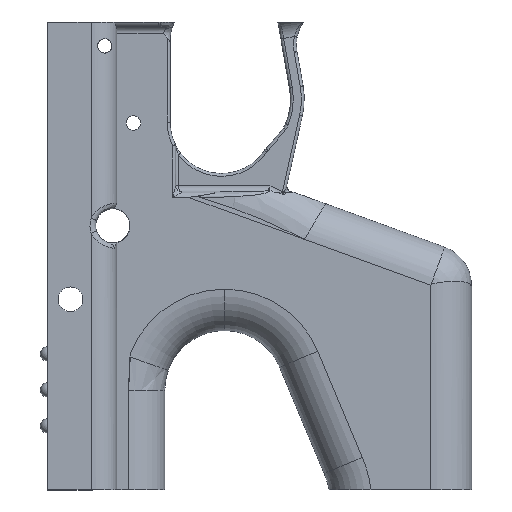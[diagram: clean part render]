
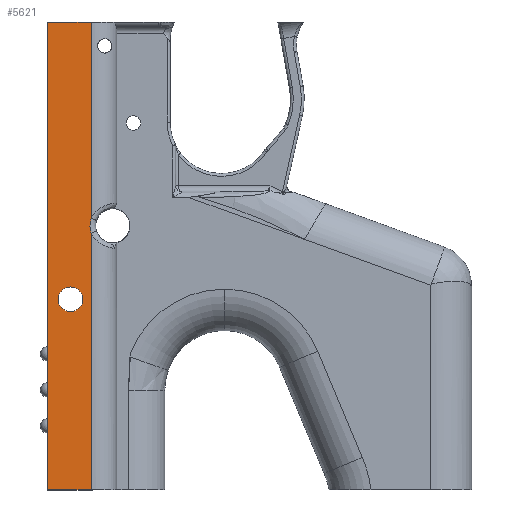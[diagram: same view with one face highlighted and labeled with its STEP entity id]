
A CAD part, left-side view. The second image highlights one B-rep face of the part: STEP entity #5621.
In plain terms, the highlighted planar face has unit normal (-1, 0, 0).
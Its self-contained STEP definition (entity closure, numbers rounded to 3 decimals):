
#21 = VECTOR ( 'NONE', #8800, 1000. ) ;
#68 = EDGE_CURVE ( 'NONE', #7060, #8073, #7952, .T. ) ;
#124 = DIRECTION ( 'NONE',  ( 0., 1., 0. ) ) ;
#207 = DIRECTION ( 'NONE',  ( -1., 0., 0. ) ) ;
#479 = CARTESIAN_POINT ( 'NONE',  ( 4.253, 33.602, 77.663 ) ) ;
#769 = CIRCLE ( 'NONE', #2056, 3.429 ) ;
#933 = VERTEX_POINT ( 'NONE', #3870 ) ;
#952 = CARTESIAN_POINT ( 'NONE',  ( 4.253, 33.602, -52.337 ) ) ;
#1042 = ORIENTED_EDGE ( 'NONE', *, *, #3121, .T. ) ;
#1100 = ORIENTED_EDGE ( 'NONE', *, *, #10105, .F. ) ;
#1214 = ORIENTED_EDGE ( 'NONE', *, *, #10980, .F. ) ;
#1591 = ORIENTED_EDGE ( 'NONE', *, *, #2117, .F. ) ;
#1662 = VERTEX_POINT ( 'NONE', #5119 ) ;
#1721 = CIRCLE ( 'NONE', #8557, 3.429 ) ;
#1729 = CARTESIAN_POINT ( 'NONE',  ( 4.253, 33.602, -52.337 ) ) ;
#1735 = EDGE_CURVE ( 'NONE', #11558, #3343, #9408, .T. ) ;
#2056 = AXIS2_PLACEMENT_3D ( 'NONE', #4003, #10663, #5003 ) ;
#2109 = LINE ( 'NONE', #952, #11608 ) ;
#2117 = EDGE_CURVE ( 'NONE', #1662, #4378, #1721, .T. ) ;
#2332 = AXIS2_PLACEMENT_3D ( 'NONE', #10855, #207, #7182 ) ;
#2620 = CARTESIAN_POINT ( 'NONE',  ( 4.253, 33.602, 19.005 ) ) ;
#2871 = VERTEX_POINT ( 'NONE', #2992 ) ;
#2992 = CARTESIAN_POINT ( 'NONE',  ( 4.253, 45.721, -52.337 ) ) ;
#3102 = EDGE_CURVE ( 'NONE', #7060, #2871, #2109, .T. ) ;
#3121 = EDGE_CURVE ( 'NONE', #8073, #933, #10884, .T. ) ;
#3182 = EDGE_CURVE ( 'NONE', #933, #11558, #9022, .T. ) ;
#3343 = VERTEX_POINT ( 'NONE', #8854 ) ;
#3510 = CARTESIAN_POINT ( 'NONE',  ( 4.253, 33.602, 19.005 ) ) ;
#3870 = CARTESIAN_POINT ( 'NONE',  ( 4.253, 33.602, 23.07 ) ) ;
#4003 = CARTESIAN_POINT ( 'NONE',  ( 4.253, 39.359, 0.641 ) ) ;
#4378 = VERTEX_POINT ( 'NONE', #8688 ) ;
#4851 = CARTESIAN_POINT ( 'NONE',  ( 4.253, 33.602, 77.663 ) ) ;
#5003 = DIRECTION ( 'NONE',  ( 0., 0., 1. ) ) ;
#5119 = CARTESIAN_POINT ( 'NONE',  ( 4.253, 39.359, -2.788 ) ) ;
#5426 = DIRECTION ( 'NONE',  ( 0., 0., 1. ) ) ;
#5463 = ORIENTED_EDGE ( 'NONE', *, *, #3182, .T. ) ;
#5621 = ADVANCED_FACE ( 'NONE', ( #10233, #7756 ), #9979, .T. ) ;
#6222 = CARTESIAN_POINT ( 'NONE',  ( 4.253, 33.602, 141.062 ) ) ;
#6896 = ORIENTED_EDGE ( 'NONE', *, *, #68, .T. ) ;
#7060 = VERTEX_POINT ( 'NONE', #1729 ) ;
#7182 = DIRECTION ( 'NONE',  ( 0., 0., 1. ) ) ;
#7756 = FACE_BOUND ( 'NONE', #11450, .T. ) ;
#7952 = LINE ( 'NONE', #9132, #21 ) ;
#8073 = VERTEX_POINT ( 'NONE', #2620 ) ;
#8542 = DIRECTION ( 'NONE',  ( 0., 0., 1. ) ) ;
#8553 = DIRECTION ( 'NONE',  ( -1., 0., 0. ) ) ;
#8555 = CARTESIAN_POINT ( 'NONE',  ( 4.253, 39.359, 0.641 ) ) ;
#8557 = AXIS2_PLACEMENT_3D ( 'NONE', #8555, #8553, #8542 ) ;
#8688 = CARTESIAN_POINT ( 'NONE',  ( 4.253, 39.359, 4.07 ) ) ;
#8705 = CARTESIAN_POINT ( 'NONE',  ( 4.253, 45.721, 162.566 ) ) ;
#8800 = DIRECTION ( 'NONE',  ( 0., 0., 1. ) ) ;
#8854 = CARTESIAN_POINT ( 'NONE',  ( 4.253, 45.721, 77.663 ) ) ;
#8971 = EDGE_LOOP ( 'NONE', ( #10931, #6896, #1042, #5463, #9931, #1214 ) ) ;
#9022 = LINE ( 'NONE', #6222, #11117 ) ;
#9132 = CARTESIAN_POINT ( 'NONE',  ( 4.253, 33.602, 141.062 ) ) ;
#9408 = LINE ( 'NONE', #4851, #11431 ) ;
#9931 = ORIENTED_EDGE ( 'NONE', *, *, #1735, .T. ) ;
#9979 = PLANE ( 'NONE',  #2332 ) ;
#10105 = EDGE_CURVE ( 'NONE', #4378, #1662, #769, .T. ) ;
#10233 = FACE_OUTER_BOUND ( 'NONE', #8971, .T. ) ;
#10497 = DIRECTION ( 'NONE',  ( 0., 0., 1. ) ) ;
#10565 = DIRECTION ( 'NONE',  ( 0., 1., 0. ) ) ;
#10648 = VECTOR ( 'NONE', #10497, 1000. ) ;
#10663 = DIRECTION ( 'NONE',  ( -1., 0., 0. ) ) ;
#10855 = CARTESIAN_POINT ( 'NONE',  ( 4.253, 33.602, 141.062 ) ) ;
#10884 = B_SPLINE_CURVE_WITH_KNOTS ( 'NONE', 3,
 ( #3510, #11804, #11771, #11738, #11703, #11668 ),
 .UNSPECIFIED., .F., .F.,
 ( 4, 2, 4 ),
 ( 0., 0.5, 1. ),
 .UNSPECIFIED. ) ;
#10905 = LINE ( 'NONE', #8705, #10648 ) ;
#10931 = ORIENTED_EDGE ( 'NONE', *, *, #3102, .F. ) ;
#10980 = EDGE_CURVE ( 'NONE', #2871, #3343, #10905, .T. ) ;
#11117 = VECTOR ( 'NONE', #5426, 1000. ) ;
#11431 = VECTOR ( 'NONE', #10565, 1000. ) ;
#11450 = EDGE_LOOP ( 'NONE', ( #1100, #1591 ) ) ;
#11558 = VERTEX_POINT ( 'NONE', #479 ) ;
#11608 = VECTOR ( 'NONE', #124, 1000. ) ;
#11668 = CARTESIAN_POINT ( 'NONE',  ( 4.253, 33.602, 23.07 ) ) ;
#11703 = CARTESIAN_POINT ( 'NONE',  ( 4.253, 33.824, 22.41 ) ) ;
#11738 = CARTESIAN_POINT ( 'NONE',  ( 4.253, 33.936, 21.733 ) ) ;
#11771 = CARTESIAN_POINT ( 'NONE',  ( 4.253, 33.936, 20.342 ) ) ;
#11804 = CARTESIAN_POINT ( 'NONE',  ( 4.253, 33.824, 19.664 ) ) ;
